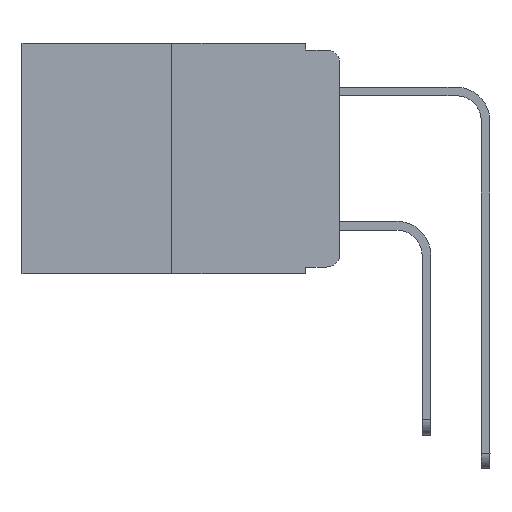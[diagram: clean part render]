
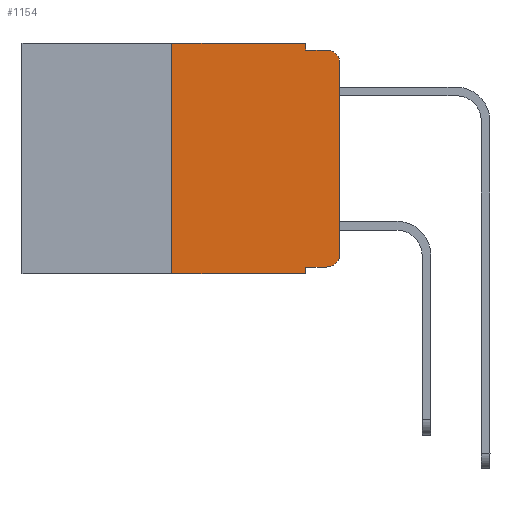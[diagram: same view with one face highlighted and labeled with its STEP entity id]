
A CAD part, left-side view. The second image highlights one B-rep face of the part: STEP entity #1154.
In plain terms, the highlighted planar face has unit normal (-1, 0, 0).
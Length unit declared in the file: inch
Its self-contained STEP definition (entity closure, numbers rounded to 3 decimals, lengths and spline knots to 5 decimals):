
#182 = DIRECTION ( 'NONE',  ( 0., -1., 0. ) ) ;
#404 = EDGE_CURVE ( 'NONE', #15666, #11844, #1528, .T. ) ;
#557 = CARTESIAN_POINT ( 'NONE',  ( 0., 0.02, -0.03 ) ) ;
#628 = EDGE_LOOP ( 'NONE', ( #8567, #14470, #12128, #10112, #8560, #10762, #12387, #13326, #14288, #5334 ) ) ;
#1036 = LINE ( 'NONE', #9214, #13815 ) ;
#1125 = CARTESIAN_POINT ( 'NONE',  ( 0., 0.051, -0.01 ) ) ;
#1154 = ADVANCED_FACE ( 'NONE', ( #4857 ), #11601, .F. ) ;
#1395 = EDGE_CURVE ( 'NONE', #13893, #7086, #8678, .T. ) ;
#1501 = CARTESIAN_POINT ( 'NONE',  ( 0., 0.051, 0. ) ) ;
#1528 = LINE ( 'NONE', #6897, #6697 ) ;
#1874 = DIRECTION ( 'NONE',  ( 0., 0., -1. ) ) ;
#2929 = DIRECTION ( 'NONE',  ( 0., -1., 0. ) ) ;
#3134 = VECTOR ( 'NONE', #8958, 39.37008 ) ;
#3225 = CARTESIAN_POINT ( 'NONE',  ( 0., 0.25, 0. ) ) ;
#3304 = LINE ( 'NONE', #3225, #14782 ) ;
#3809 = CARTESIAN_POINT ( 'NONE',  ( 0., 0.051, -0.01 ) ) ;
#4296 = EDGE_CURVE ( 'NONE', #11844, #14559, #12406, .T. ) ;
#4373 = VERTEX_POINT ( 'NONE', #8797 ) ;
#4658 = EDGE_CURVE ( 'NONE', #13713, #11884, #1036, .T. ) ;
#4808 = VECTOR ( 'NONE', #9662, 39.37008 ) ;
#4857 = FACE_OUTER_BOUND ( 'NONE', #628, .T. ) ;
#5024 = LINE ( 'NONE', #1125, #3134 ) ;
#5107 = DIRECTION ( 'NONE',  ( 0., 0., -1. ) ) ;
#5334 = ORIENTED_EDGE ( 'NONE', *, *, #8284, .T. ) ;
#5885 = EDGE_CURVE ( 'NONE', #14559, #13266, #5024, .T. ) ;
#6155 = EDGE_CURVE ( 'NONE', #13713, #12004, #13783, .T. ) ;
#6697 = VECTOR ( 'NONE', #2929, 39.37008 ) ;
#6897 = CARTESIAN_POINT ( 'NONE',  ( 0., 0.473, 0. ) ) ;
#6994 = CIRCLE ( 'NONE', #9235, 0.02 ) ;
#7086 = VERTEX_POINT ( 'NONE', #7300 ) ;
#7300 = CARTESIAN_POINT ( 'NONE',  ( 0., 0., -0.03 ) ) ;
#7924 = VECTOR ( 'NONE', #12639, 39.37008 ) ;
#8284 = EDGE_CURVE ( 'NONE', #12004, #13893, #13595, .T. ) ;
#8426 = CARTESIAN_POINT ( 'NONE',  ( 0., 0.25, 0. ) ) ;
#8560 = ORIENTED_EDGE ( 'NONE', *, *, #404, .F. ) ;
#8567 = ORIENTED_EDGE ( 'NONE', *, *, #1395, .T. ) ;
#8678 = LINE ( 'NONE', #10139, #14150 ) ;
#8797 = CARTESIAN_POINT ( 'NONE',  ( 0., 0.25, -0.343 ) ) ;
#8958 = DIRECTION ( 'NONE',  ( 0., -1., 0. ) ) ;
#9159 = CARTESIAN_POINT ( 'NONE',  ( 0., 0.02, -0.313 ) ) ;
#9214 = CARTESIAN_POINT ( 'NONE',  ( 0., 0.051, 0. ) ) ;
#9235 = AXIS2_PLACEMENT_3D ( 'NONE', #557, #13846, #1874 ) ;
#9237 = CARTESIAN_POINT ( 'NONE',  ( 0., 0.051, 0. ) ) ;
#9434 = AXIS2_PLACEMENT_3D ( 'NONE', #10186, #10267, #15646 ) ;
#9662 = DIRECTION ( 'NONE',  ( 0., 0., -1. ) ) ;
#10112 = ORIENTED_EDGE ( 'NONE', *, *, #4296, .F. ) ;
#10139 = CARTESIAN_POINT ( 'NONE',  ( 0., 0., 0. ) ) ;
#10186 = CARTESIAN_POINT ( 'NONE',  ( 0., 0.473, 0. ) ) ;
#10267 = DIRECTION ( 'NONE',  ( 1., 0., 0. ) ) ;
#10440 = CARTESIAN_POINT ( 'NONE',  ( 0., 0.051, -0.333 ) ) ;
#10669 = EDGE_CURVE ( 'NONE', #4373, #15666, #3304, .T. ) ;
#10762 = ORIENTED_EDGE ( 'NONE', *, *, #10669, .F. ) ;
#10884 = CARTESIAN_POINT ( 'NONE',  ( 0., 0.051, -0.343 ) ) ;
#10893 = CARTESIAN_POINT ( 'NONE',  ( 0., 0.473, -0.343 ) ) ;
#11051 = CARTESIAN_POINT ( 'NONE',  ( 0., 0.02, -0.333 ) ) ;
#11061 = LINE ( 'NONE', #10893, #17167 ) ;
#11601 = PLANE ( 'NONE',  #9434 ) ;
#11798 = CARTESIAN_POINT ( 'NONE',  ( 0., 0.02, -0.01 ) ) ;
#11844 = VERTEX_POINT ( 'NONE', #9237 ) ;
#11884 = VERTEX_POINT ( 'NONE', #10884 ) ;
#12004 = VERTEX_POINT ( 'NONE', #11051 ) ;
#12128 = ORIENTED_EDGE ( 'NONE', *, *, #5885, .F. ) ;
#12387 = ORIENTED_EDGE ( 'NONE', *, *, #16400, .T. ) ;
#12406 = LINE ( 'NONE', #1501, #4808 ) ;
#12639 = DIRECTION ( 'NONE',  ( 0., -1., 0. ) ) ;
#12714 = DIRECTION ( 'NONE',  ( 0., 0., 1. ) ) ;
#12748 = AXIS2_PLACEMENT_3D ( 'NONE', #9159, #13031, #13297 ) ;
#13031 = DIRECTION ( 'NONE',  ( -1., 0., 0. ) ) ;
#13266 = VERTEX_POINT ( 'NONE', #11798 ) ;
#13297 = DIRECTION ( 'NONE',  ( 0., 0., -1. ) ) ;
#13326 = ORIENTED_EDGE ( 'NONE', *, *, #4658, .F. ) ;
#13595 = CIRCLE ( 'NONE', #12748, 0.02 ) ;
#13713 = VERTEX_POINT ( 'NONE', #10440 ) ;
#13783 = LINE ( 'NONE', #13871, #7924 ) ;
#13815 = VECTOR ( 'NONE', #5107, 39.37008 ) ;
#13846 = DIRECTION ( 'NONE',  ( -1., 0., 0. ) ) ;
#13871 = CARTESIAN_POINT ( 'NONE',  ( 0., 0.051, -0.333 ) ) ;
#13879 = CARTESIAN_POINT ( 'NONE',  ( 0., 0., -0.313 ) ) ;
#13893 = VERTEX_POINT ( 'NONE', #13879 ) ;
#14150 = VECTOR ( 'NONE', #15184, 39.37008 ) ;
#14288 = ORIENTED_EDGE ( 'NONE', *, *, #6155, .T. ) ;
#14470 = ORIENTED_EDGE ( 'NONE', *, *, #16815, .T. ) ;
#14559 = VERTEX_POINT ( 'NONE', #3809 ) ;
#14782 = VECTOR ( 'NONE', #12714, 39.37008 ) ;
#15184 = DIRECTION ( 'NONE',  ( 0., 0., 1. ) ) ;
#15646 = DIRECTION ( 'NONE',  ( 0., 0., -1. ) ) ;
#15666 = VERTEX_POINT ( 'NONE', #8426 ) ;
#16400 = EDGE_CURVE ( 'NONE', #4373, #11884, #11061, .T. ) ;
#16815 = EDGE_CURVE ( 'NONE', #7086, #13266, #6994, .T. ) ;
#17167 = VECTOR ( 'NONE', #182, 39.37008 ) ;
